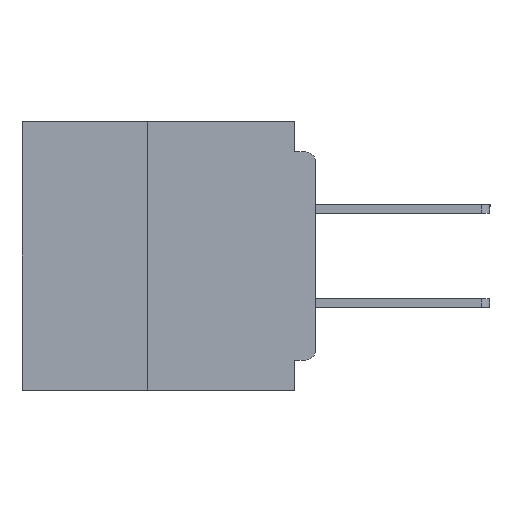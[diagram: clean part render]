
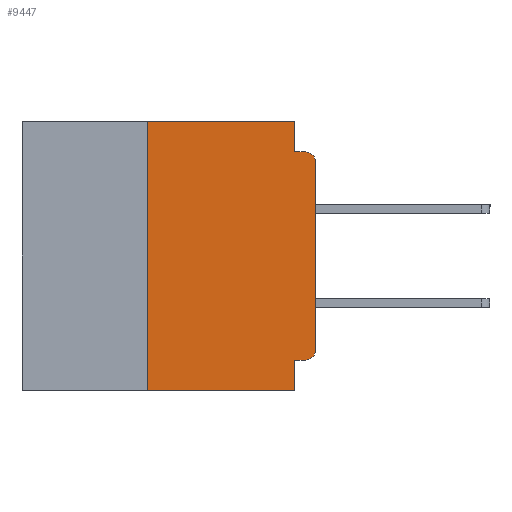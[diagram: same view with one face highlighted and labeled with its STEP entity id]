
A CAD part, left-side view. The second image highlights one B-rep face of the part: STEP entity #9447.
In plain terms, the highlighted planar face has unit normal (-1, 0, 0).
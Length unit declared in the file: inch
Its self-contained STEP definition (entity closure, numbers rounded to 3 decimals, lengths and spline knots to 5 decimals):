
#326 = AXIS2_PLACEMENT_3D ( 'NONE', #22654, #51206, #26736 ) ;
#866 = DIRECTION ( 'NONE',  ( 0., 0., -1. ) ) ;
#1425 = ORIENTED_EDGE ( 'NONE', *, *, #8367, .F. ) ;
#1598 = VECTOR ( 'NONE', #42504, 39.37008 ) ;
#1606 = VERTEX_POINT ( 'NONE', #18609 ) ;
#1830 = ORIENTED_EDGE ( 'NONE', *, *, #36454, .T. ) ;
#2001 = VERTEX_POINT ( 'NONE', #12473 ) ;
#2869 = VECTOR ( 'NONE', #29169, 39.37008 ) ;
#4389 = VERTEX_POINT ( 'NONE', #12064 ) ;
#4757 = LINE ( 'NONE', #15008, #34919 ) ;
#5659 = CARTESIAN_POINT ( 'NONE',  ( 0., 0.031, -0.045 ) ) ;
#8367 = EDGE_CURVE ( 'NONE', #50919, #49899, #25241, .T. ) ;
#8871 = ORIENTED_EDGE ( 'NONE', *, *, #41405, .T. ) ;
#9447 = ADVANCED_FACE ( 'NONE', ( #47497 ), #49994, .F. ) ;
#10220 = CARTESIAN_POINT ( 'NONE',  ( 0., 0.031, -0.4 ) ) ;
#11319 = VERTEX_POINT ( 'NONE', #22845 ) ;
#12046 = DIRECTION ( 'NONE',  ( -1., 0., 0. ) ) ;
#12064 = CARTESIAN_POINT ( 'NONE',  ( 0., 0.25, -0.4 ) ) ;
#12473 = CARTESIAN_POINT ( 'NONE',  ( 0., 0.015, -0.355 ) ) ;
#12983 = CARTESIAN_POINT ( 'NONE',  ( 0., 0., -0.06 ) ) ;
#13136 = CARTESIAN_POINT ( 'NONE',  ( 0., 0., 0. ) ) ;
#13753 = CARTESIAN_POINT ( 'NONE',  ( 0., 0., -0.045 ) ) ;
#13927 = EDGE_CURVE ( 'NONE', #11319, #48184, #50221, .T. ) ;
#14457 = ORIENTED_EDGE ( 'NONE', *, *, #18601, .F. ) ;
#14770 = EDGE_CURVE ( 'NONE', #45563, #1606, #29664, .T. ) ;
#15008 = CARTESIAN_POINT ( 'NONE',  ( 0., 0., -0.355 ) ) ;
#17146 = ORIENTED_EDGE ( 'NONE', *, *, #52808, .F. ) ;
#17293 = CARTESIAN_POINT ( 'NONE',  ( 0., 0.437, 0. ) ) ;
#17709 = ORIENTED_EDGE ( 'NONE', *, *, #14770, .T. ) ;
#18601 = EDGE_CURVE ( 'NONE', #40735, #11319, #36037, .T. ) ;
#18609 = CARTESIAN_POINT ( 'NONE',  ( 0., 0.015, -0.045 ) ) ;
#19133 = DIRECTION ( 'NONE',  ( 0., 1., 0. ) ) ;
#21656 = CARTESIAN_POINT ( 'NONE',  ( 0., 0.031, 0. ) ) ;
#22290 = LINE ( 'NONE', #51824, #42718 ) ;
#22596 = DIRECTION ( 'NONE',  ( 0., 0., -1. ) ) ;
#22654 = CARTESIAN_POINT ( 'NONE',  ( 0., 0.015, -0.06 ) ) ;
#22845 = CARTESIAN_POINT ( 'NONE',  ( 0., 0.031, 0. ) ) ;
#25241 = LINE ( 'NONE', #10220, #45692 ) ;
#25499 = DIRECTION ( 'NONE',  ( 1., 0., 0. ) ) ;
#25567 = DIRECTION ( 'NONE',  ( 0., 0., -1. ) ) ;
#25959 = EDGE_CURVE ( 'NONE', #48184, #1606, #45225, .T. ) ;
#26435 = VECTOR ( 'NONE', #32183, 39.37008 ) ;
#26736 = DIRECTION ( 'NONE',  ( 0., 0., -1. ) ) ;
#28186 = CARTESIAN_POINT ( 'NONE',  ( 0., 0.25, 0. ) ) ;
#29169 = DIRECTION ( 'NONE',  ( 0., -1., 0. ) ) ;
#29566 = DIRECTION ( 'NONE',  ( 0., 0., 1. ) ) ;
#29664 = CIRCLE ( 'NONE', #326, 0.015 ) ;
#30622 = VERTEX_POINT ( 'NONE', #33012 ) ;
#31593 = LINE ( 'NONE', #13136, #41208 ) ;
#32183 = DIRECTION ( 'NONE',  ( 0., -1., 0. ) ) ;
#32465 = ORIENTED_EDGE ( 'NONE', *, *, #25959, .F. ) ;
#33012 = CARTESIAN_POINT ( 'NONE',  ( 0., 0., -0.34 ) ) ;
#33270 = CARTESIAN_POINT ( 'NONE',  ( 0., 0.437, -0.4 ) ) ;
#34919 = VECTOR ( 'NONE', #19133, 39.37008 ) ;
#35620 = LINE ( 'NONE', #33270, #2869 ) ;
#36037 = LINE ( 'NONE', #36126, #26435 ) ;
#36126 = CARTESIAN_POINT ( 'NONE',  ( 0., 0.437, 0. ) ) ;
#36454 = EDGE_CURVE ( 'NONE', #30622, #45563, #31593, .T. ) ;
#36525 = CARTESIAN_POINT ( 'NONE',  ( 0., 0.015, -0.34 ) ) ;
#37689 = ORIENTED_EDGE ( 'NONE', *, *, #48031, .T. ) ;
#38062 = VECTOR ( 'NONE', #25567, 39.37008 ) ;
#40070 = CIRCLE ( 'NONE', #43093, 0.015 ) ;
#40653 = DIRECTION ( 'NONE',  ( 0., 0., -1. ) ) ;
#40735 = VERTEX_POINT ( 'NONE', #28186 ) ;
#41208 = VECTOR ( 'NONE', #29566, 39.37008 ) ;
#41405 = EDGE_CURVE ( 'NONE', #2001, #30622, #40070, .T. ) ;
#42504 = DIRECTION ( 'NONE',  ( 0., -1., 0. ) ) ;
#42718 = VECTOR ( 'NONE', #47897, 39.37008 ) ;
#43093 = AXIS2_PLACEMENT_3D ( 'NONE', #36525, #12046, #40653 ) ;
#45084 = CARTESIAN_POINT ( 'NONE',  ( 0., 0.031, -0.4 ) ) ;
#45225 = LINE ( 'NONE', #13753, #1598 ) ;
#45563 = VERTEX_POINT ( 'NONE', #12983 ) ;
#45692 = VECTOR ( 'NONE', #22596, 39.37008 ) ;
#45895 = ORIENTED_EDGE ( 'NONE', *, *, #46543, .F. ) ;
#46543 = EDGE_CURVE ( 'NONE', #4389, #40735, #22290, .T. ) ;
#47056 = EDGE_LOOP ( 'NONE', ( #1830, #17709, #32465, #49831, #14457, #45895, #37689, #1425, #17146, #8871 ) ) ;
#47497 = FACE_OUTER_BOUND ( 'NONE', #47056, .T. ) ;
#47897 = DIRECTION ( 'NONE',  ( 0., 0., 1. ) ) ;
#48031 = EDGE_CURVE ( 'NONE', #4389, #49899, #35620, .T. ) ;
#48184 = VERTEX_POINT ( 'NONE', #5659 ) ;
#49220 = AXIS2_PLACEMENT_3D ( 'NONE', #17293, #25499, #866 ) ;
#49831 = ORIENTED_EDGE ( 'NONE', *, *, #13927, .F. ) ;
#49899 = VERTEX_POINT ( 'NONE', #45084 ) ;
#49994 = PLANE ( 'NONE',  #49220 ) ;
#50221 = LINE ( 'NONE', #21656, #38062 ) ;
#50919 = VERTEX_POINT ( 'NONE', #51592 ) ;
#51206 = DIRECTION ( 'NONE',  ( -1., 0., 0. ) ) ;
#51592 = CARTESIAN_POINT ( 'NONE',  ( 0., 0.031, -0.355 ) ) ;
#51824 = CARTESIAN_POINT ( 'NONE',  ( 0., 0.25, -0.4 ) ) ;
#52808 = EDGE_CURVE ( 'NONE', #2001, #50919, #4757, .T. ) ;
